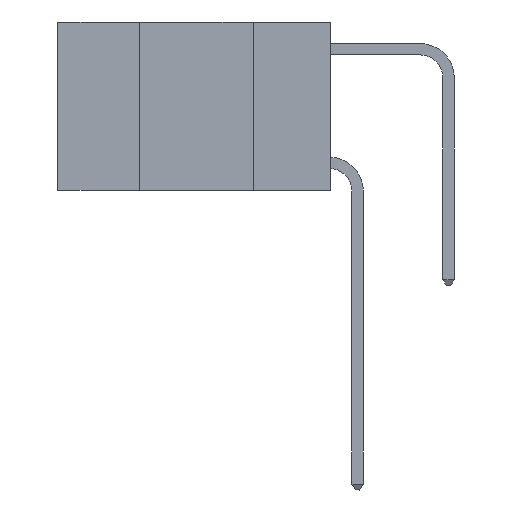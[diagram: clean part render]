
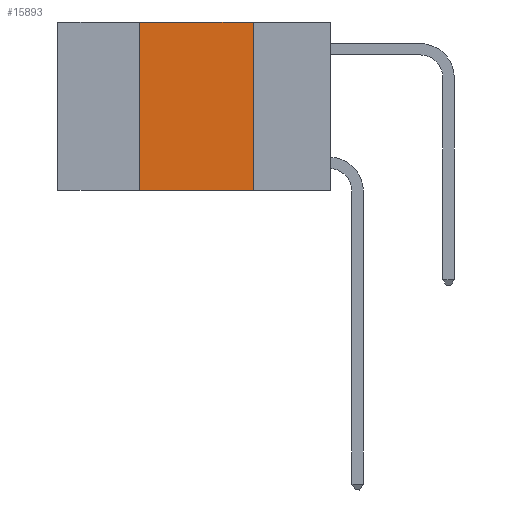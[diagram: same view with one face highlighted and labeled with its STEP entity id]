
A CAD part, left-side view. The second image highlights one B-rep face of the part: STEP entity #15893.
In plain terms, the highlighted planar face has unit normal (-1, 0, 0).
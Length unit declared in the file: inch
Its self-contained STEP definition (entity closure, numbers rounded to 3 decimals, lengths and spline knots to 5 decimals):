
#104 = CARTESIAN_POINT ( 'NONE',  ( 0., 0.42, 0. ) ) ;
#502 = DIRECTION ( 'NONE',  ( 0., -1., 0. ) ) ;
#852 = VECTOR ( 'NONE', #6865, 39.37008 ) ;
#1126 = EDGE_CURVE ( 'NONE', #1997, #4804, #11586, .T. ) ;
#1526 = DIRECTION ( 'NONE',  ( 0., 0., -1. ) ) ;
#1982 = CARTESIAN_POINT ( 'NONE',  ( 0., 0.6, -0.37 ) ) ;
#1997 = VERTEX_POINT ( 'NONE', #10135 ) ;
#3002 = DIRECTION ( 'NONE',  ( 0., 0., -1. ) ) ;
#3457 = CARTESIAN_POINT ( 'NONE',  ( 0., 0.6, 0. ) ) ;
#3461 = EDGE_CURVE ( 'NONE', #17192, #11692, #12773, .T. ) ;
#4804 = VERTEX_POINT ( 'NONE', #11432 ) ;
#5135 = FACE_OUTER_BOUND ( 'NONE', #14837, .T. ) ;
#5727 = EDGE_CURVE ( 'NONE', #11692, #1997, #8870, .T. ) ;
#6865 = DIRECTION ( 'NONE',  ( 0., 0., 1. ) ) ;
#6991 = CARTESIAN_POINT ( 'NONE',  ( 0., 0.17, 0. ) ) ;
#7179 = EDGE_CURVE ( 'NONE', #17192, #4804, #15902, .T. ) ;
#7290 = CARTESIAN_POINT ( 'NONE',  ( 0., 0.6, 0. ) ) ;
#7334 = VECTOR ( 'NONE', #3002, 39.37008 ) ;
#8683 = PLANE ( 'NONE',  #14867 ) ;
#8870 = LINE ( 'NONE', #3457, #9326 ) ;
#9326 = VECTOR ( 'NONE', #16225, 39.37008 ) ;
#9972 = CARTESIAN_POINT ( 'NONE',  ( 0., 0.42, -0.37 ) ) ;
#10135 = CARTESIAN_POINT ( 'NONE',  ( 0., 0.17, 0. ) ) ;
#10138 = DIRECTION ( 'NONE',  ( 1., 0., 0. ) ) ;
#10193 = CARTESIAN_POINT ( 'NONE',  ( 0., 0.42, 0. ) ) ;
#11432 = CARTESIAN_POINT ( 'NONE',  ( 0., 0.17, -0.37 ) ) ;
#11586 = LINE ( 'NONE', #6991, #7334 ) ;
#11692 = VERTEX_POINT ( 'NONE', #10193 ) ;
#12773 = LINE ( 'NONE', #104, #852 ) ;
#14837 = EDGE_LOOP ( 'NONE', ( #16329, #16817, #17117, #17450 ) ) ;
#14867 = AXIS2_PLACEMENT_3D ( 'NONE', #7290, #10138, #1526 ) ;
#15464 = VECTOR ( 'NONE', #502, 39.37008 ) ;
#15893 = ADVANCED_FACE ( 'NONE', ( #5135 ), #8683, .F. ) ;
#15902 = LINE ( 'NONE', #1982, #15464 ) ;
#16225 = DIRECTION ( 'NONE',  ( 0., -1., 0. ) ) ;
#16329 = ORIENTED_EDGE ( 'NONE', *, *, #1126, .F. ) ;
#16817 = ORIENTED_EDGE ( 'NONE', *, *, #5727, .F. ) ;
#17117 = ORIENTED_EDGE ( 'NONE', *, *, #3461, .F. ) ;
#17192 = VERTEX_POINT ( 'NONE', #9972 ) ;
#17450 = ORIENTED_EDGE ( 'NONE', *, *, #7179, .T. ) ;
